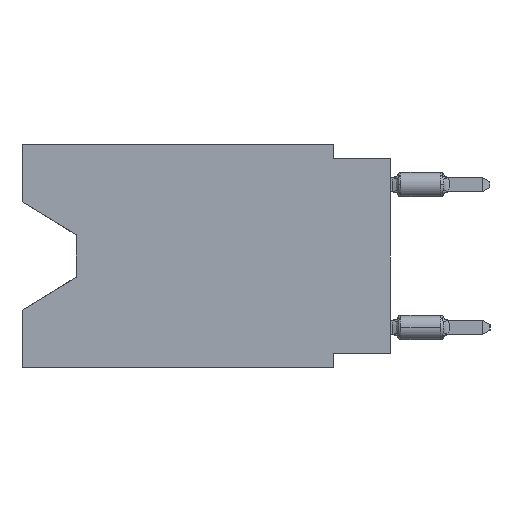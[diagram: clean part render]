
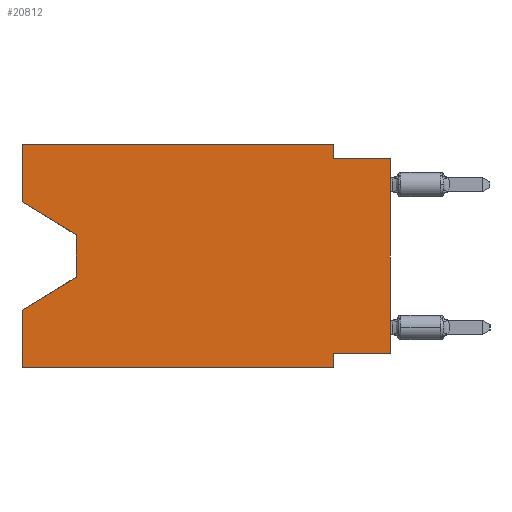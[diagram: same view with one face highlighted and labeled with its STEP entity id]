
A CAD part, left-side view. The second image highlights one B-rep face of the part: STEP entity #20812.
In plain terms, the highlighted planar face has unit normal (-1, 0, 0).
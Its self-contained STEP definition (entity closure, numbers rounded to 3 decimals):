
#260 = CARTESIAN_POINT ( 'NONE',  ( 0., 16.383, 0. ) ) ;
#435 = LINE ( 'NONE', #2730, #7766 ) ;
#450 = CARTESIAN_POINT ( 'NONE',  ( 0., 2.54, 0. ) ) ;
#699 = CARTESIAN_POINT ( 'NONE',  ( 0., 2.54, -9.906 ) ) ;
#1284 = LINE ( 'NONE', #14783, #7214 ) ;
#1301 = DIRECTION ( 'NONE',  ( 1., 0., 0. ) ) ;
#1317 = ORIENTED_EDGE ( 'NONE', *, *, #8963, .T. ) ;
#1855 = VECTOR ( 'NONE', #20369, 1000. ) ;
#2045 = LINE ( 'NONE', #699, #20631 ) ;
#2730 = CARTESIAN_POINT ( 'NONE',  ( 0., 0., -0.635 ) ) ;
#2749 = EDGE_CURVE ( 'NONE', #16376, #20733, #14172, .T. ) ;
#3069 = CARTESIAN_POINT ( 'NONE',  ( 0., 2.54, -9.906 ) ) ;
#4879 = DIRECTION ( 'NONE',  ( 0., 0.855, -0.519 ) ) ;
#4999 = ORIENTED_EDGE ( 'NONE', *, *, #12933, .F. ) ;
#5023 = CARTESIAN_POINT ( 'NONE',  ( 0., 0., -9.271 ) ) ;
#5117 = CARTESIAN_POINT ( 'NONE',  ( 0., 13.97, -5.893 ) ) ;
#5144 = EDGE_CURVE ( 'NONE', #20733, #12687, #27211, .T. ) ;
#5605 = ORIENTED_EDGE ( 'NONE', *, *, #17256, .T. ) ;
#6125 = CARTESIAN_POINT ( 'NONE',  ( 0., 16.383, -9.906 ) ) ;
#6592 = ORIENTED_EDGE ( 'NONE', *, *, #2749, .F. ) ;
#7085 = EDGE_CURVE ( 'NONE', #11571, #15711, #20107, .T. ) ;
#7157 = EDGE_CURVE ( 'NONE', #17569, #21504, #16227, .T. ) ;
#7214 = VECTOR ( 'NONE', #10475, 1000. ) ;
#7523 = CARTESIAN_POINT ( 'NONE',  ( 0., 2.54, 0. ) ) ;
#7700 = CARTESIAN_POINT ( 'NONE',  ( 0., 13.97, -4.013 ) ) ;
#7766 = VECTOR ( 'NONE', #13356, 1000. ) ;
#8139 = DIRECTION ( 'NONE',  ( 0., -1., 0. ) ) ;
#8185 = LINE ( 'NONE', #18956, #19259 ) ;
#8464 = LINE ( 'NONE', #17229, #16772 ) ;
#8521 = ORIENTED_EDGE ( 'NONE', *, *, #11953, .T. ) ;
#8719 = CARTESIAN_POINT ( 'NONE',  ( 0., 0., 0. ) ) ;
#8963 = EDGE_CURVE ( 'NONE', #17911, #27893, #1284, .T. ) ;
#8972 = AXIS2_PLACEMENT_3D ( 'NONE', #20835, #1301, #11932 ) ;
#9547 = VECTOR ( 'NONE', #23077, 1000. ) ;
#10475 = DIRECTION ( 'NONE',  ( 0., -0.855, -0.519 ) ) ;
#10622 = ORIENTED_EDGE ( 'NONE', *, *, #7085, .F. ) ;
#11190 = ORIENTED_EDGE ( 'NONE', *, *, #18186, .F. ) ;
#11571 = VERTEX_POINT ( 'NONE', #14972 ) ;
#11932 = DIRECTION ( 'NONE',  ( 0., 0., -1. ) ) ;
#11953 = EDGE_CURVE ( 'NONE', #20221, #15140, #8464, .T. ) ;
#12092 = CARTESIAN_POINT ( 'NONE',  ( 0., 2.54, -0.635 ) ) ;
#12427 = CARTESIAN_POINT ( 'NONE',  ( 0., 16.383, 0. ) ) ;
#12597 = DIRECTION ( 'NONE',  ( 0., 0., 1. ) ) ;
#12687 = VERTEX_POINT ( 'NONE', #12092 ) ;
#12789 = VECTOR ( 'NONE', #12597, 1000. ) ;
#12933 = EDGE_CURVE ( 'NONE', #20221, #21504, #26978, .T. ) ;
#13356 = DIRECTION ( 'NONE',  ( 0., -1., 0. ) ) ;
#13641 = CARTESIAN_POINT ( 'NONE',  ( 0., 13.97, -4.013 ) ) ;
#14172 = LINE ( 'NONE', #12427, #19113 ) ;
#14471 = VECTOR ( 'NONE', #4879, 1000. ) ;
#14783 = CARTESIAN_POINT ( 'NONE',  ( 0., 16.383, -2.546 ) ) ;
#14972 = CARTESIAN_POINT ( 'NONE',  ( 0., 0., -9.271 ) ) ;
#15140 = VERTEX_POINT ( 'NONE', #3069 ) ;
#15711 = VERTEX_POINT ( 'NONE', #25439 ) ;
#15773 = VERTEX_POINT ( 'NONE', #26698 ) ;
#16227 = LINE ( 'NONE', #24567, #14471 ) ;
#16376 = VERTEX_POINT ( 'NONE', #19293 ) ;
#16772 = VECTOR ( 'NONE', #25997, 1000. ) ;
#17229 = CARTESIAN_POINT ( 'NONE',  ( 0., 16.383, -9.906 ) ) ;
#17256 = EDGE_CURVE ( 'NONE', #11571, #15773, #23827, .T. ) ;
#17569 = VERTEX_POINT ( 'NONE', #5117 ) ;
#17650 = EDGE_LOOP ( 'NONE', ( #1317, #20119, #21303, #4999, #8521, #11190, #10622, #5605, #22142, #23677, #6592, #18696 ) ) ;
#17911 = VERTEX_POINT ( 'NONE', #25335 ) ;
#17954 = DIRECTION ( 'NONE',  ( 0., 1., 0. ) ) ;
#18186 = EDGE_CURVE ( 'NONE', #15711, #15140, #2045, .T. ) ;
#18696 = ORIENTED_EDGE ( 'NONE', *, *, #24202, .F. ) ;
#18698 = PLANE ( 'NONE',  #8972 ) ;
#18956 = CARTESIAN_POINT ( 'NONE',  ( 0., 16.383, 0. ) ) ;
#19113 = VECTOR ( 'NONE', #8139, 1000. ) ;
#19259 = VECTOR ( 'NONE', #27712, 1000. ) ;
#19293 = CARTESIAN_POINT ( 'NONE',  ( 0., 16.383, 0. ) ) ;
#19636 = CARTESIAN_POINT ( 'NONE',  ( 0., 16.383, -7.36 ) ) ;
#20107 = LINE ( 'NONE', #5023, #23195 ) ;
#20119 = ORIENTED_EDGE ( 'NONE', *, *, #22876, .T. ) ;
#20221 = VERTEX_POINT ( 'NONE', #6125 ) ;
#20369 = DIRECTION ( 'NONE',  ( 0., 0., 1. ) ) ;
#20631 = VECTOR ( 'NONE', #26840, 1000. ) ;
#20733 = VERTEX_POINT ( 'NONE', #450 ) ;
#20812 = ADVANCED_FACE ( 'NONE', ( #22709 ), #18698, .F. ) ;
#20835 = CARTESIAN_POINT ( 'NONE',  ( 0., 16.383, 0. ) ) ;
#21242 = VECTOR ( 'NONE', #25061, 1000. ) ;
#21303 = ORIENTED_EDGE ( 'NONE', *, *, #7157, .T. ) ;
#21504 = VERTEX_POINT ( 'NONE', #19636 ) ;
#22142 = ORIENTED_EDGE ( 'NONE', *, *, #27954, .F. ) ;
#22645 = LINE ( 'NONE', #7700, #9547 ) ;
#22709 = FACE_OUTER_BOUND ( 'NONE', #17650, .T. ) ;
#22876 = EDGE_CURVE ( 'NONE', #27893, #17569, #22645, .T. ) ;
#23077 = DIRECTION ( 'NONE',  ( 0., 0., -1. ) ) ;
#23195 = VECTOR ( 'NONE', #17954, 1000. ) ;
#23677 = ORIENTED_EDGE ( 'NONE', *, *, #5144, .F. ) ;
#23827 = LINE ( 'NONE', #8719, #12789 ) ;
#24202 = EDGE_CURVE ( 'NONE', #17911, #16376, #8185, .T. ) ;
#24567 = CARTESIAN_POINT ( 'NONE',  ( 0., 13.97, -5.893 ) ) ;
#25061 = DIRECTION ( 'NONE',  ( 0., 0., -1. ) ) ;
#25335 = CARTESIAN_POINT ( 'NONE',  ( 0., 16.383, -2.546 ) ) ;
#25439 = CARTESIAN_POINT ( 'NONE',  ( 0., 2.54, -9.271 ) ) ;
#25997 = DIRECTION ( 'NONE',  ( 0., -1., 0. ) ) ;
#26698 = CARTESIAN_POINT ( 'NONE',  ( 0., 0., -0.635 ) ) ;
#26840 = DIRECTION ( 'NONE',  ( 0., 0., -1. ) ) ;
#26978 = LINE ( 'NONE', #260, #1855 ) ;
#27211 = LINE ( 'NONE', #7523, #21242 ) ;
#27712 = DIRECTION ( 'NONE',  ( 0., 0., 1. ) ) ;
#27893 = VERTEX_POINT ( 'NONE', #13641 ) ;
#27954 = EDGE_CURVE ( 'NONE', #12687, #15773, #435, .T. ) ;
